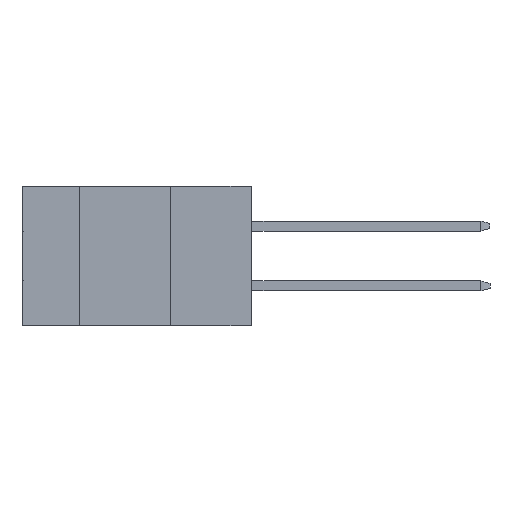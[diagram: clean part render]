
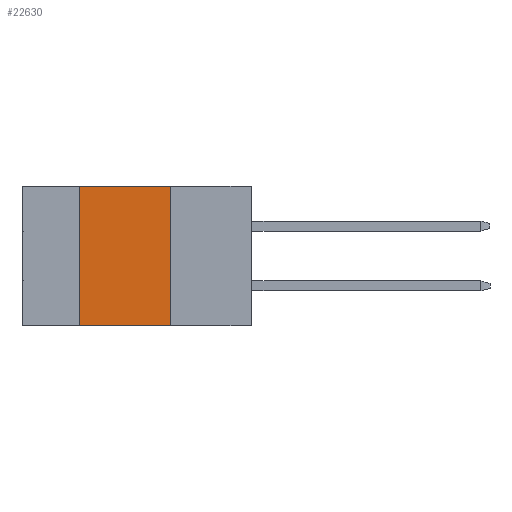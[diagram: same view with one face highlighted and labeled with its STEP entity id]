
A CAD part, left-side view. The second image highlights one B-rep face of the part: STEP entity #22630.
In plain terms, the highlighted planar face has unit normal (-1, 0, 0).
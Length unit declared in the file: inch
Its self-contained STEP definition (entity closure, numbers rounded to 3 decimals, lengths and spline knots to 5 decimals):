
#275 = VERTEX_POINT ( 'NONE', #2768 ) ;
#1644 = DIRECTION ( 'NONE',  ( 1., 0., 0. ) ) ;
#2207 = EDGE_CURVE ( 'NONE', #275, #4938, #8536, .T. ) ;
#2768 = CARTESIAN_POINT ( 'NONE',  ( 0., 0.54, 0. ) ) ;
#3053 = CARTESIAN_POINT ( 'NONE',  ( 0., 0.254, 0. ) ) ;
#3170 = ORIENTED_EDGE ( 'NONE', *, *, #9748, .T. ) ;
#3457 = DIRECTION ( 'NONE',  ( 0., 0., 1. ) ) ;
#3467 = VECTOR ( 'NONE', #19342, 39.37008 ) ;
#4768 = EDGE_CURVE ( 'NONE', #8175, #275, #8899, .T. ) ;
#4938 = VERTEX_POINT ( 'NONE', #3053 ) ;
#5958 = CARTESIAN_POINT ( 'NONE',  ( 0., 0.54, -0.437 ) ) ;
#6006 = CARTESIAN_POINT ( 'NONE',  ( 0., 0.254, -0.437 ) ) ;
#7094 = AXIS2_PLACEMENT_3D ( 'NONE', #12269, #1644, #20883 ) ;
#7533 = DIRECTION ( 'NONE',  ( 0., 0., -1. ) ) ;
#8144 = VECTOR ( 'NONE', #7533, 39.37008 ) ;
#8175 = VERTEX_POINT ( 'NONE', #9640 ) ;
#8536 = LINE ( 'NONE', #14097, #3467 ) ;
#8899 = LINE ( 'NONE', #5958, #20490 ) ;
#9125 = CARTESIAN_POINT ( 'NONE',  ( 0., 0.72, -0.437 ) ) ;
#9640 = CARTESIAN_POINT ( 'NONE',  ( 0., 0.54, -0.437 ) ) ;
#9748 = EDGE_CURVE ( 'NONE', #8175, #14612, #12586, .T. ) ;
#9893 = ORIENTED_EDGE ( 'NONE', *, *, #4768, .F. ) ;
#10541 = PLANE ( 'NONE',  #7094 ) ;
#11300 = ORIENTED_EDGE ( 'NONE', *, *, #2207, .F. ) ;
#12269 = CARTESIAN_POINT ( 'NONE',  ( 0., 0.72, 0. ) ) ;
#12586 = LINE ( 'NONE', #9125, #20365 ) ;
#12830 = LINE ( 'NONE', #6006, #8144 ) ;
#12861 = EDGE_LOOP ( 'NONE', ( #18935, #11300, #9893, #3170 ) ) ;
#14097 = CARTESIAN_POINT ( 'NONE',  ( 0., 0.72, 0. ) ) ;
#14587 = CARTESIAN_POINT ( 'NONE',  ( 0., 0.254, -0.437 ) ) ;
#14612 = VERTEX_POINT ( 'NONE', #14587 ) ;
#16145 = DIRECTION ( 'NONE',  ( 0., -1., 0. ) ) ;
#18935 = ORIENTED_EDGE ( 'NONE', *, *, #21540, .F. ) ;
#19342 = DIRECTION ( 'NONE',  ( 0., -1., 0. ) ) ;
#20365 = VECTOR ( 'NONE', #16145, 39.37008 ) ;
#20490 = VECTOR ( 'NONE', #3457, 39.37008 ) ;
#20759 = FACE_OUTER_BOUND ( 'NONE', #12861, .T. ) ;
#20883 = DIRECTION ( 'NONE',  ( 0., 0., -1. ) ) ;
#21540 = EDGE_CURVE ( 'NONE', #4938, #14612, #12830, .T. ) ;
#22630 = ADVANCED_FACE ( 'NONE', ( #20759 ), #10541, .F. ) ;
